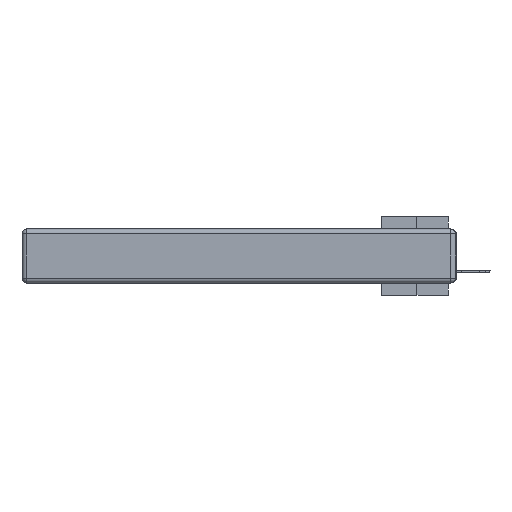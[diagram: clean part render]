
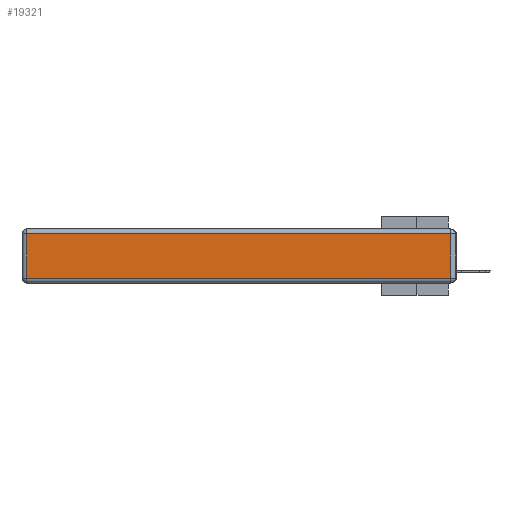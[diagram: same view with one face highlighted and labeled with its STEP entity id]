
A CAD part, left-side view. The second image highlights one B-rep face of the part: STEP entity #19321.
In plain terms, the highlighted planar face has unit normal (-1, 0, 0).
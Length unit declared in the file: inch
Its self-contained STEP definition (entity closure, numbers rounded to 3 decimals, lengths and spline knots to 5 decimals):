
#205 = VERTEX_POINT ( 'NONE', #1161 ) ;
#608 = EDGE_LOOP ( 'NONE', ( #28245, #2752, #4485, #27195 ) ) ;
#1161 = CARTESIAN_POINT ( 'NONE',  ( 0., 2.72, -0.313 ) ) ;
#1296 = EDGE_CURVE ( 'NONE', #26291, #205, #2031, .T. ) ;
#1500 = DIRECTION ( 'NONE',  ( 0., 0., -1. ) ) ;
#2031 = LINE ( 'NONE', #17026, #27109 ) ;
#2752 = ORIENTED_EDGE ( 'NONE', *, *, #14933, .T. ) ;
#3847 = CARTESIAN_POINT ( 'NONE',  ( 0., 0.03, -0.313 ) ) ;
#4026 = DIRECTION ( 'NONE',  ( 0., 1., 0. ) ) ;
#4485 = ORIENTED_EDGE ( 'NONE', *, *, #32802, .T. ) ;
#4615 = AXIS2_PLACEMENT_3D ( 'NONE', #17620, #12517, #9972 ) ;
#5648 = LINE ( 'NONE', #30197, #20725 ) ;
#6672 = CARTESIAN_POINT ( 'NONE',  ( 0., 2.75, -0.03 ) ) ;
#8757 = LINE ( 'NONE', #28479, #27851 ) ;
#9659 = VECTOR ( 'NONE', #4026, 39.37008 ) ;
#9743 = FACE_OUTER_BOUND ( 'NONE', #608, .T. ) ;
#9972 = DIRECTION ( 'NONE',  ( 0., 0., 1. ) ) ;
#12408 = PLANE ( 'NONE',  #4615 ) ;
#12517 = DIRECTION ( 'NONE',  ( -1., 0., 0. ) ) ;
#14933 = EDGE_CURVE ( 'NONE', #19692, #22221, #8757, .T. ) ;
#17026 = CARTESIAN_POINT ( 'NONE',  ( 0., 2.72, -0.343 ) ) ;
#17620 = CARTESIAN_POINT ( 'NONE',  ( 0., 0., -0.343 ) ) ;
#19321 = ADVANCED_FACE ( 'NONE', ( #9743 ), #12408, .T. ) ;
#19692 = VERTEX_POINT ( 'NONE', #3847 ) ;
#20466 = DIRECTION ( 'NONE',  ( 0., -1., 0. ) ) ;
#20545 = CARTESIAN_POINT ( 'NONE',  ( 0., 0.03, -0.03 ) ) ;
#20725 = VECTOR ( 'NONE', #20466, 39.37008 ) ;
#22221 = VERTEX_POINT ( 'NONE', #20545 ) ;
#23008 = DIRECTION ( 'NONE',  ( 0., 0., 1. ) ) ;
#26291 = VERTEX_POINT ( 'NONE', #27273 ) ;
#27109 = VECTOR ( 'NONE', #1500, 39.37008 ) ;
#27190 = LINE ( 'NONE', #6672, #9659 ) ;
#27195 = ORIENTED_EDGE ( 'NONE', *, *, #1296, .T. ) ;
#27273 = CARTESIAN_POINT ( 'NONE',  ( 0., 2.72, -0.03 ) ) ;
#27851 = VECTOR ( 'NONE', #23008, 39.37008 ) ;
#28245 = ORIENTED_EDGE ( 'NONE', *, *, #28658, .T. ) ;
#28479 = CARTESIAN_POINT ( 'NONE',  ( 0., 0.03, -0.343 ) ) ;
#28658 = EDGE_CURVE ( 'NONE', #205, #19692, #5648, .T. ) ;
#30197 = CARTESIAN_POINT ( 'NONE',  ( 0., 0., -0.313 ) ) ;
#32802 = EDGE_CURVE ( 'NONE', #22221, #26291, #27190, .T. ) ;
